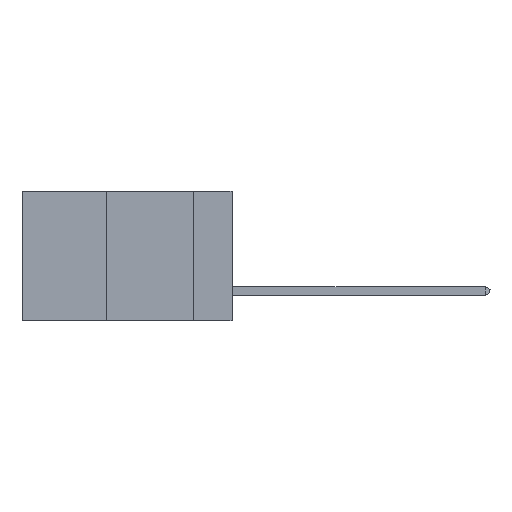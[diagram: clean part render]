
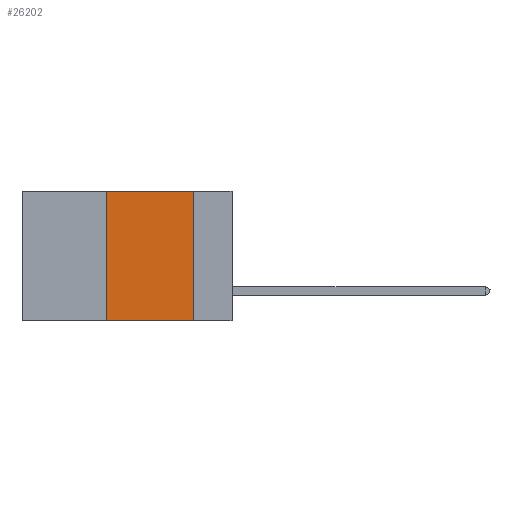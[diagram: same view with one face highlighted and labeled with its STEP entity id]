
A CAD part, left-side view. The second image highlights one B-rep face of the part: STEP entity #26202.
In plain terms, the highlighted planar face has unit normal (-1, 0, 0).
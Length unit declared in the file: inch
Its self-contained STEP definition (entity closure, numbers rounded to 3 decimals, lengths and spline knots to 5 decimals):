
#159 = ORIENTED_EDGE ( 'NONE', *, *, #27887, .F. ) ;
#1560 = CARTESIAN_POINT ( 'NONE',  ( 0., 0.6, -0.37 ) ) ;
#2099 = EDGE_LOOP ( 'NONE', ( #11193, #159, #3601, #15069 ) ) ;
#2526 = DIRECTION ( 'NONE',  ( 0., 0., -1. ) ) ;
#3535 = VECTOR ( 'NONE', #2526, 39.37008 ) ;
#3601 = ORIENTED_EDGE ( 'NONE', *, *, #21324, .F. ) ;
#3669 = VECTOR ( 'NONE', #9758, 39.37008 ) ;
#5979 = CARTESIAN_POINT ( 'NONE',  ( 0., 0.11, -0.37 ) ) ;
#6026 = VECTOR ( 'NONE', #15742, 39.37008 ) ;
#8293 = VERTEX_POINT ( 'NONE', #5979 ) ;
#9758 = DIRECTION ( 'NONE',  ( 0., 0., 1. ) ) ;
#10272 = DIRECTION ( 'NONE',  ( 0., -1., 0. ) ) ;
#11193 = ORIENTED_EDGE ( 'NONE', *, *, #23179, .F. ) ;
#11216 = LINE ( 'NONE', #1560, #6026 ) ;
#11708 = CARTESIAN_POINT ( 'NONE',  ( 0., 0.36, 0. ) ) ;
#12271 = VERTEX_POINT ( 'NONE', #31888 ) ;
#12575 = PLANE ( 'NONE',  #35755 ) ;
#13050 = CARTESIAN_POINT ( 'NONE',  ( 0., 0.6, 0. ) ) ;
#13544 = VERTEX_POINT ( 'NONE', #21594 ) ;
#13924 = EDGE_CURVE ( 'NONE', #12271, #8293, #11216, .T. ) ;
#15069 = ORIENTED_EDGE ( 'NONE', *, *, #13924, .T. ) ;
#15742 = DIRECTION ( 'NONE',  ( 0., -1., 0. ) ) ;
#18416 = LINE ( 'NONE', #31532, #3669 ) ;
#20605 = DIRECTION ( 'NONE',  ( 1., 0., 0. ) ) ;
#21324 = EDGE_CURVE ( 'NONE', #12271, #25912, #18416, .T. ) ;
#21594 = CARTESIAN_POINT ( 'NONE',  ( 0., 0.11, 0. ) ) ;
#22106 = VECTOR ( 'NONE', #10272, 39.37008 ) ;
#23179 = EDGE_CURVE ( 'NONE', #13544, #8293, #24369, .T. ) ;
#24369 = LINE ( 'NONE', #27910, #3535 ) ;
#25912 = VERTEX_POINT ( 'NONE', #11708 ) ;
#26202 = ADVANCED_FACE ( 'NONE', ( #31257 ), #12575, .F. ) ;
#27887 = EDGE_CURVE ( 'NONE', #25912, #13544, #30267, .T. ) ;
#27910 = CARTESIAN_POINT ( 'NONE',  ( 0., 0.11, 0. ) ) ;
#30267 = LINE ( 'NONE', #13050, #22106 ) ;
#31257 = FACE_OUTER_BOUND ( 'NONE', #2099, .T. ) ;
#31532 = CARTESIAN_POINT ( 'NONE',  ( 0., 0.36, 0. ) ) ;
#31888 = CARTESIAN_POINT ( 'NONE',  ( 0., 0.36, -0.37 ) ) ;
#31947 = DIRECTION ( 'NONE',  ( 0., 0., -1. ) ) ;
#34383 = CARTESIAN_POINT ( 'NONE',  ( 0., 0.6, 0. ) ) ;
#35755 = AXIS2_PLACEMENT_3D ( 'NONE', #34383, #20605, #31947 ) ;
